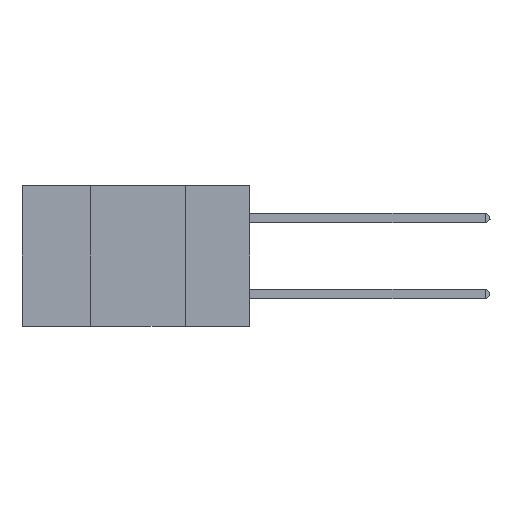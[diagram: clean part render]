
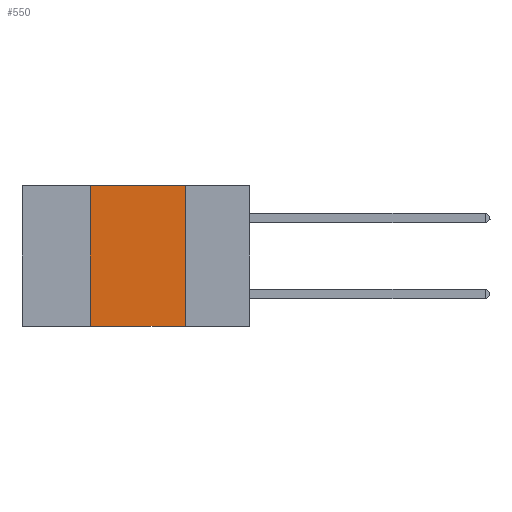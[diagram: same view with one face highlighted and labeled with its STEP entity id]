
A CAD part, left-side view. The second image highlights one B-rep face of the part: STEP entity #550.
In plain terms, the highlighted planar face has unit normal (-1, 0, 0).
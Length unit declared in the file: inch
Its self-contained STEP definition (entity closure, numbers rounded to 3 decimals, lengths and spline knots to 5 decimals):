
#64 = VERTEX_POINT ( 'NONE', #2814 ) ;
#167 = EDGE_CURVE ( 'NONE', #13995, #64, #5793, .T. ) ;
#550 = ADVANCED_FACE ( 'NONE', ( #11989 ), #5360, .F. ) ;
#1916 = LINE ( 'NONE', #12484, #13670 ) ;
#1972 = EDGE_CURVE ( 'NONE', #13995, #3103, #9311, .T. ) ;
#2510 = ORIENTED_EDGE ( 'NONE', *, *, #1972, .F. ) ;
#2633 = CARTESIAN_POINT ( 'NONE',  ( 0., 0.6, 0. ) ) ;
#2644 = CARTESIAN_POINT ( 'NONE',  ( 0., 0.42, 0. ) ) ;
#2814 = CARTESIAN_POINT ( 'NONE',  ( 0., 0.17, -0.37 ) ) ;
#3103 = VERTEX_POINT ( 'NONE', #16611 ) ;
#3776 = VECTOR ( 'NONE', #16127, 39.37008 ) ;
#4124 = DIRECTION ( 'NONE',  ( 0., -1., 0. ) ) ;
#4196 = DIRECTION ( 'NONE',  ( 0., 0., -1. ) ) ;
#4622 = CARTESIAN_POINT ( 'NONE',  ( 0., 0.42, -0.37 ) ) ;
#5351 = AXIS2_PLACEMENT_3D ( 'NONE', #13132, #11907, #13476 ) ;
#5360 = PLANE ( 'NONE',  #5351 ) ;
#5793 = LINE ( 'NONE', #13747, #15717 ) ;
#5862 = EDGE_CURVE ( 'NONE', #8196, #64, #1916, .T. ) ;
#5883 = DIRECTION ( 'NONE',  ( 0., -1., 0. ) ) ;
#6840 = LINE ( 'NONE', #2633, #9490 ) ;
#7382 = CARTESIAN_POINT ( 'NONE',  ( 0., 0.17, 0. ) ) ;
#8196 = VERTEX_POINT ( 'NONE', #7382 ) ;
#9311 = LINE ( 'NONE', #2644, #3776 ) ;
#9490 = VECTOR ( 'NONE', #4124, 39.37008 ) ;
#11041 = EDGE_LOOP ( 'NONE', ( #15798, #14968, #2510, #16378 ) ) ;
#11117 = EDGE_CURVE ( 'NONE', #3103, #8196, #6840, .T. ) ;
#11907 = DIRECTION ( 'NONE',  ( 1., 0., 0. ) ) ;
#11989 = FACE_OUTER_BOUND ( 'NONE', #11041, .T. ) ;
#12484 = CARTESIAN_POINT ( 'NONE',  ( 0., 0.17, 0. ) ) ;
#13132 = CARTESIAN_POINT ( 'NONE',  ( 0., 0.6, 0. ) ) ;
#13476 = DIRECTION ( 'NONE',  ( 0., 0., -1. ) ) ;
#13670 = VECTOR ( 'NONE', #4196, 39.37008 ) ;
#13747 = CARTESIAN_POINT ( 'NONE',  ( 0., 0.6, -0.37 ) ) ;
#13995 = VERTEX_POINT ( 'NONE', #4622 ) ;
#14968 = ORIENTED_EDGE ( 'NONE', *, *, #11117, .F. ) ;
#15717 = VECTOR ( 'NONE', #5883, 39.37008 ) ;
#15798 = ORIENTED_EDGE ( 'NONE', *, *, #5862, .F. ) ;
#16127 = DIRECTION ( 'NONE',  ( 0., 0., 1. ) ) ;
#16378 = ORIENTED_EDGE ( 'NONE', *, *, #167, .T. ) ;
#16611 = CARTESIAN_POINT ( 'NONE',  ( 0., 0.42, 0. ) ) ;
